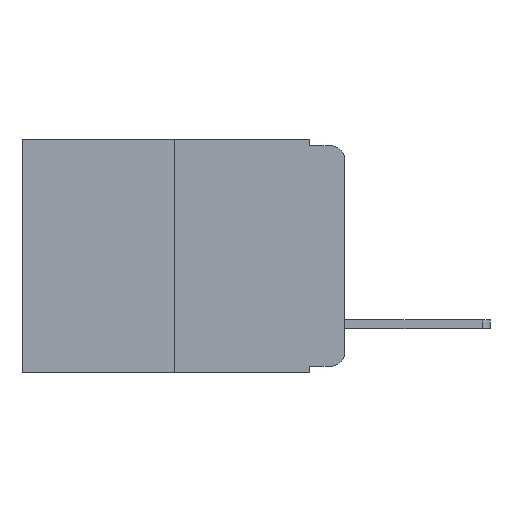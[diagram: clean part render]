
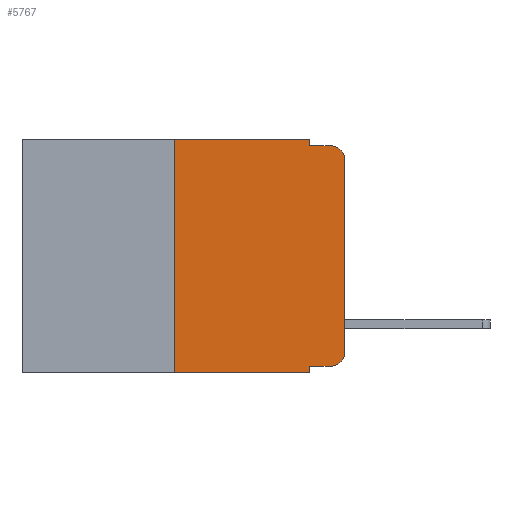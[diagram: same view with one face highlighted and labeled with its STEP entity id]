
A CAD part, left-side view. The second image highlights one B-rep face of the part: STEP entity #5767.
In plain terms, the highlighted planar face has unit normal (-1, 0, 0).
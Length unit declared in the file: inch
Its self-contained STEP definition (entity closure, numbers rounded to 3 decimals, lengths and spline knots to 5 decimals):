
#32 = DIRECTION ( 'NONE',  ( 1., 0., 0. ) ) ;
#89 = DIRECTION ( 'NONE',  ( 0., -1., 0. ) ) ;
#691 = VERTEX_POINT ( 'NONE', #1744 ) ;
#857 = DIRECTION ( 'NONE',  ( -1., 0., 0. ) ) ;
#1034 = VERTEX_POINT ( 'NONE', #3608 ) ;
#1203 = CARTESIAN_POINT ( 'NONE',  ( 0., 0.25, -0.343 ) ) ;
#1239 = EDGE_CURVE ( 'NONE', #3092, #6566, #7342, .T. ) ;
#1378 = DIRECTION ( 'NONE',  ( 0., -1., 0. ) ) ;
#1418 = FACE_OUTER_BOUND ( 'NONE', #6979, .T. ) ;
#1609 = DIRECTION ( 'NONE',  ( 0., 0., -1. ) ) ;
#1628 = ORIENTED_EDGE ( 'NONE', *, *, #7337, .F. ) ;
#1744 = CARTESIAN_POINT ( 'NONE',  ( 0., 0.02, -0.01 ) ) ;
#2016 = VERTEX_POINT ( 'NONE', #10021 ) ;
#2525 = ORIENTED_EDGE ( 'NONE', *, *, #7986, .T. ) ;
#2676 = CARTESIAN_POINT ( 'NONE',  ( 0., 0., -0.03 ) ) ;
#3001 = AXIS2_PLACEMENT_3D ( 'NONE', #5636, #32, #6528 ) ;
#3092 = VERTEX_POINT ( 'NONE', #5378 ) ;
#3105 = EDGE_CURVE ( 'NONE', #4624, #1034, #10371, .T. ) ;
#3412 = VECTOR ( 'NONE', #7447, 39.37008 ) ;
#3529 = ORIENTED_EDGE ( 'NONE', *, *, #1239, .F. ) ;
#3608 = CARTESIAN_POINT ( 'NONE',  ( 0., 0.051, -0.343 ) ) ;
#3625 = VERTEX_POINT ( 'NONE', #7331 ) ;
#3744 = LINE ( 'NONE', #4185, #10269 ) ;
#3777 = EDGE_CURVE ( 'NONE', #6566, #691, #10225, .T. ) ;
#3851 = LINE ( 'NONE', #7880, #8194 ) ;
#3856 = VECTOR ( 'NONE', #5492, 39.37008 ) ;
#4185 = CARTESIAN_POINT ( 'NONE',  ( 0., 0., 0. ) ) ;
#4457 = CARTESIAN_POINT ( 'NONE',  ( 0., 0.02, -0.03 ) ) ;
#4511 = ORIENTED_EDGE ( 'NONE', *, *, #6890, .T. ) ;
#4624 = VERTEX_POINT ( 'NONE', #1203 ) ;
#4990 = VECTOR ( 'NONE', #6352, 39.37008 ) ;
#5028 = CARTESIAN_POINT ( 'NONE',  ( 0., 0.25, 0. ) ) ;
#5145 = VERTEX_POINT ( 'NONE', #6538 ) ;
#5374 = DIRECTION ( 'NONE',  ( 0., 0., -1. ) ) ;
#5378 = CARTESIAN_POINT ( 'NONE',  ( 0., 0.051, 0. ) ) ;
#5404 = LINE ( 'NONE', #9276, #7697 ) ;
#5492 = DIRECTION ( 'NONE',  ( 0., -1., 0. ) ) ;
#5636 = CARTESIAN_POINT ( 'NONE',  ( 0., 0.473, 0. ) ) ;
#5767 = ADVANCED_FACE ( 'NONE', ( #1418 ), #11325, .F. ) ;
#6303 = EDGE_CURVE ( 'NONE', #7008, #3625, #8239, .T. ) ;
#6352 = DIRECTION ( 'NONE',  ( 0., 0., -1. ) ) ;
#6370 = CARTESIAN_POINT ( 'NONE',  ( 0., 0.02, -0.313 ) ) ;
#6483 = ORIENTED_EDGE ( 'NONE', *, *, #3105, .T. ) ;
#6528 = DIRECTION ( 'NONE',  ( 0., 0., -1. ) ) ;
#6538 = CARTESIAN_POINT ( 'NONE',  ( 0., 0.25, 0. ) ) ;
#6566 = VERTEX_POINT ( 'NONE', #10022 ) ;
#6579 = CARTESIAN_POINT ( 'NONE',  ( 0., 0.473, 0. ) ) ;
#6841 = DIRECTION ( 'NONE',  ( 0., 0., 1. ) ) ;
#6890 = EDGE_CURVE ( 'NONE', #3625, #8997, #3744, .T. ) ;
#6979 = EDGE_LOOP ( 'NONE', ( #4511, #9047, #9555, #3529, #8164, #1628, #6483, #8938, #2525, #9441 ) ) ;
#7008 = VERTEX_POINT ( 'NONE', #11066 ) ;
#7235 = DIRECTION ( 'NONE',  ( 0., 0., -1. ) ) ;
#7260 = CARTESIAN_POINT ( 'NONE',  ( 0., 0.051, -0.01 ) ) ;
#7331 = CARTESIAN_POINT ( 'NONE',  ( 0., 0., -0.313 ) ) ;
#7337 = EDGE_CURVE ( 'NONE', #4624, #5145, #9993, .T. ) ;
#7342 = LINE ( 'NONE', #8728, #4990 ) ;
#7447 = DIRECTION ( 'NONE',  ( 0., -1., 0. ) ) ;
#7697 = VECTOR ( 'NONE', #1378, 39.37008 ) ;
#7847 = VECTOR ( 'NONE', #10859, 39.37008 ) ;
#7880 = CARTESIAN_POINT ( 'NONE',  ( 0., 0.051, 0. ) ) ;
#7986 = EDGE_CURVE ( 'NONE', #2016, #7008, #5404, .T. ) ;
#8164 = ORIENTED_EDGE ( 'NONE', *, *, #9092, .F. ) ;
#8194 = VECTOR ( 'NONE', #1609, 39.37008 ) ;
#8239 = CIRCLE ( 'NONE', #8609, 0.02 ) ;
#8609 = AXIS2_PLACEMENT_3D ( 'NONE', #6370, #857, #7235 ) ;
#8728 = CARTESIAN_POINT ( 'NONE',  ( 0., 0.051, 0. ) ) ;
#8938 = ORIENTED_EDGE ( 'NONE', *, *, #10053, .F. ) ;
#8962 = EDGE_CURVE ( 'NONE', #8997, #691, #9113, .T. ) ;
#8997 = VERTEX_POINT ( 'NONE', #2676 ) ;
#9047 = ORIENTED_EDGE ( 'NONE', *, *, #8962, .T. ) ;
#9092 = EDGE_CURVE ( 'NONE', #5145, #3092, #10267, .T. ) ;
#9113 = CIRCLE ( 'NONE', #10406, 0.02 ) ;
#9276 = CARTESIAN_POINT ( 'NONE',  ( 0., 0.051, -0.333 ) ) ;
#9441 = ORIENTED_EDGE ( 'NONE', *, *, #6303, .T. ) ;
#9555 = ORIENTED_EDGE ( 'NONE', *, *, #3777, .F. ) ;
#9610 = CARTESIAN_POINT ( 'NONE',  ( 0., 0.473, -0.343 ) ) ;
#9753 = VECTOR ( 'NONE', #89, 39.37008 ) ;
#9993 = LINE ( 'NONE', #5028, #7847 ) ;
#10021 = CARTESIAN_POINT ( 'NONE',  ( 0., 0.051, -0.333 ) ) ;
#10022 = CARTESIAN_POINT ( 'NONE',  ( 0., 0.051, -0.01 ) ) ;
#10053 = EDGE_CURVE ( 'NONE', #2016, #1034, #3851, .T. ) ;
#10225 = LINE ( 'NONE', #7260, #3412 ) ;
#10267 = LINE ( 'NONE', #6579, #9753 ) ;
#10269 = VECTOR ( 'NONE', #6841, 39.37008 ) ;
#10371 = LINE ( 'NONE', #9610, #3856 ) ;
#10374 = DIRECTION ( 'NONE',  ( -1., 0., 0. ) ) ;
#10406 = AXIS2_PLACEMENT_3D ( 'NONE', #4457, #10374, #5374 ) ;
#10859 = DIRECTION ( 'NONE',  ( 0., 0., 1. ) ) ;
#11066 = CARTESIAN_POINT ( 'NONE',  ( 0., 0.02, -0.333 ) ) ;
#11325 = PLANE ( 'NONE',  #3001 ) ;
